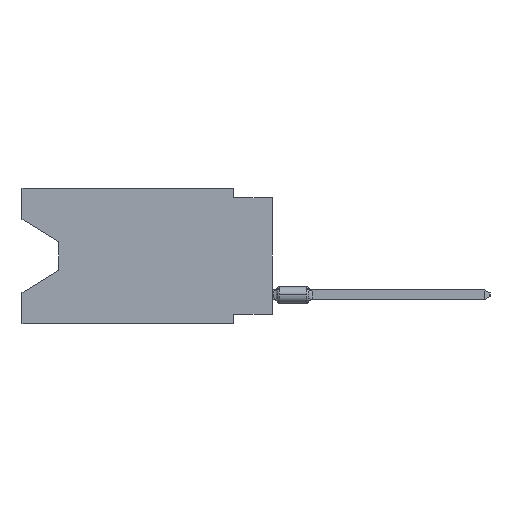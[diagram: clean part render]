
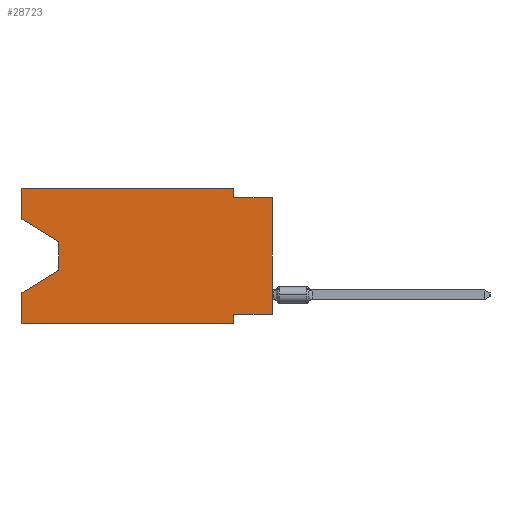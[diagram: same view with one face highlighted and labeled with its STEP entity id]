
A CAD part, left-side view. The second image highlights one B-rep face of the part: STEP entity #28723.
In plain terms, the highlighted planar face has unit normal (-1, 0, 0).
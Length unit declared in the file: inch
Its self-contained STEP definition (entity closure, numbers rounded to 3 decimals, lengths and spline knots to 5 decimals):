
#227 = CARTESIAN_POINT ( 'NONE',  ( 0., 0.55, -0.212 ) ) ;
#2391 = DIRECTION ( 'NONE',  ( 0., 0., -1. ) ) ;
#2712 = EDGE_CURVE ( 'NONE', #57532, #56211, #56468, .T. ) ;
#2886 = VERTEX_POINT ( 'NONE', #9775 ) ;
#2933 = VERTEX_POINT ( 'NONE', #9493 ) ;
#2992 = VECTOR ( 'NONE', #24589, 39.37008 ) ;
#4648 = EDGE_CURVE ( 'NONE', #56844, #14403, #43599, .T. ) ;
#4980 = LINE ( 'NONE', #18821, #54229 ) ;
#5857 = DIRECTION ( 'NONE',  ( 0., 0., -1. ) ) ;
#6178 = ORIENTED_EDGE ( 'NONE', *, *, #4648, .F. ) ;
#6564 = ORIENTED_EDGE ( 'NONE', *, *, #32936, .T. ) ;
#8254 = ORIENTED_EDGE ( 'NONE', *, *, #43584, .F. ) ;
#8475 = LINE ( 'NONE', #18488, #22472 ) ;
#8972 = VECTOR ( 'NONE', #2391, 39.37008 ) ;
#9493 = CARTESIAN_POINT ( 'NONE',  ( 0., 0.1, -0.35 ) ) ;
#9775 = CARTESIAN_POINT ( 'NONE',  ( 0., 0.55, -0.212 ) ) ;
#9918 = DIRECTION ( 'NONE',  ( 0., 0., -1. ) ) ;
#10301 = CARTESIAN_POINT ( 'NONE',  ( 0., 0.645, -0.35 ) ) ;
#11115 = VERTEX_POINT ( 'NONE', #48294 ) ;
#11259 = CARTESIAN_POINT ( 'NONE',  ( 0., 0.645, 0. ) ) ;
#12315 = DIRECTION ( 'NONE',  ( 0., 0., 1. ) ) ;
#12634 = VERTEX_POINT ( 'NONE', #15781 ) ;
#13958 = DIRECTION ( 'NONE',  ( 0., 0., 1. ) ) ;
#14261 = LINE ( 'NONE', #44655, #40225 ) ;
#14403 = VERTEX_POINT ( 'NONE', #43560 ) ;
#15482 = VERTEX_POINT ( 'NONE', #50752 ) ;
#15781 = CARTESIAN_POINT ( 'NONE',  ( 0., 0.645, -0.08025 ) ) ;
#16506 = VECTOR ( 'NONE', #22323, 39.37008 ) ;
#17319 = CARTESIAN_POINT ( 'NONE',  ( 0., 0.1, -0.35 ) ) ;
#17358 = ORIENTED_EDGE ( 'NONE', *, *, #53303, .T. ) ;
#17452 = ORIENTED_EDGE ( 'NONE', *, *, #23406, .T. ) ;
#17510 = CARTESIAN_POINT ( 'NONE',  ( 0., 0., -0.025 ) ) ;
#17907 = FACE_OUTER_BOUND ( 'NONE', #54337, .T. ) ;
#18488 = CARTESIAN_POINT ( 'NONE',  ( 0., 0.645, -0.35 ) ) ;
#18821 = CARTESIAN_POINT ( 'NONE',  ( 0., 0.1, 0. ) ) ;
#19111 = VERTEX_POINT ( 'NONE', #30902 ) ;
#19414 = CARTESIAN_POINT ( 'NONE',  ( 0., 0.645, 0. ) ) ;
#19599 = ORIENTED_EDGE ( 'NONE', *, *, #25266, .T. ) ;
#19929 = EDGE_CURVE ( 'NONE', #2886, #14403, #36800, .T. ) ;
#20009 = ORIENTED_EDGE ( 'NONE', *, *, #57315, .F. ) ;
#20077 = EDGE_CURVE ( 'NONE', #12634, #45940, #25446, .T. ) ;
#21761 = LINE ( 'NONE', #22044, #16506 ) ;
#21843 = ORIENTED_EDGE ( 'NONE', *, *, #39135, .F. ) ;
#22044 = CARTESIAN_POINT ( 'NONE',  ( 0., 0.645, -0.08025 ) ) ;
#22323 = DIRECTION ( 'NONE',  ( 0., -0.855, -0.519 ) ) ;
#22472 = VECTOR ( 'NONE', #22630, 39.37008 ) ;
#22624 = DIRECTION ( 'NONE',  ( 0., 0.855, -0.519 ) ) ;
#22630 = DIRECTION ( 'NONE',  ( 0., -1., 0. ) ) ;
#22679 = DIRECTION ( 'NONE',  ( 0., -1., 0. ) ) ;
#23406 = EDGE_CURVE ( 'NONE', #57532, #36121, #14261, .T. ) ;
#24589 = DIRECTION ( 'NONE',  ( 0., 0., 1. ) ) ;
#25266 = EDGE_CURVE ( 'NONE', #56844, #2933, #8475, .T. ) ;
#25446 = LINE ( 'NONE', #38750, #2992 ) ;
#26273 = CARTESIAN_POINT ( 'NONE',  ( 0., 0.55, -0.138 ) ) ;
#26746 = DIRECTION ( 'NONE',  ( 1., 0., 0. ) ) ;
#26839 = DIRECTION ( 'NONE',  ( 0., 0., -1. ) ) ;
#27221 = VECTOR ( 'NONE', #12315, 39.37008 ) ;
#28723 = ADVANCED_FACE ( 'NONE', ( #17907 ), #40924, .F. ) ;
#28906 = ORIENTED_EDGE ( 'NONE', *, *, #19929, .T. ) ;
#29237 = LINE ( 'NONE', #17319, #8972 ) ;
#30902 = CARTESIAN_POINT ( 'NONE',  ( 0., 0.1, -0.025 ) ) ;
#32936 = EDGE_CURVE ( 'NONE', #11115, #2886, #45154, .T. ) ;
#35523 = CARTESIAN_POINT ( 'NONE',  ( 0., 0., -0.025 ) ) ;
#35965 = VECTOR ( 'NONE', #22624, 39.37008 ) ;
#36121 = VERTEX_POINT ( 'NONE', #35523 ) ;
#36552 = ORIENTED_EDGE ( 'NONE', *, *, #51704, .F. ) ;
#36701 = CARTESIAN_POINT ( 'NONE',  ( 0., 0., -0.325 ) ) ;
#36800 = LINE ( 'NONE', #227, #35965 ) ;
#36855 = LINE ( 'NONE', #19414, #42419 ) ;
#37038 = CARTESIAN_POINT ( 'NONE',  ( 0., 0.1, -0.325 ) ) ;
#38750 = CARTESIAN_POINT ( 'NONE',  ( 0., 0.645, 0. ) ) ;
#39135 = EDGE_CURVE ( 'NONE', #56211, #2933, #29237, .T. ) ;
#40225 = VECTOR ( 'NONE', #13958, 39.37008 ) ;
#40407 = VECTOR ( 'NONE', #57326, 39.37008 ) ;
#40924 = PLANE ( 'NONE',  #53612 ) ;
#42419 = VECTOR ( 'NONE', #22679, 39.37008 ) ;
#43560 = CARTESIAN_POINT ( 'NONE',  ( 0., 0.645, -0.26975 ) ) ;
#43584 = EDGE_CURVE ( 'NONE', #45940, #15482, #36855, .T. ) ;
#43599 = LINE ( 'NONE', #48604, #27221 ) ;
#44077 = LINE ( 'NONE', #17510, #45969 ) ;
#44491 = ORIENTED_EDGE ( 'NONE', *, *, #2712, .F. ) ;
#44655 = CARTESIAN_POINT ( 'NONE',  ( 0., 0., 0. ) ) ;
#45154 = LINE ( 'NONE', #26273, #54766 ) ;
#45940 = VERTEX_POINT ( 'NONE', #11259 ) ;
#45969 = VECTOR ( 'NONE', #49105, 39.37008 ) ;
#48294 = CARTESIAN_POINT ( 'NONE',  ( 0., 0.55, -0.138 ) ) ;
#48604 = CARTESIAN_POINT ( 'NONE',  ( 0., 0.645, 0. ) ) ;
#49105 = DIRECTION ( 'NONE',  ( 0., -1., 0. ) ) ;
#49561 = ORIENTED_EDGE ( 'NONE', *, *, #20077, .F. ) ;
#50752 = CARTESIAN_POINT ( 'NONE',  ( 0., 0.1, 0. ) ) ;
#51704 = EDGE_CURVE ( 'NONE', #15482, #19111, #4980, .T. ) ;
#52033 = CARTESIAN_POINT ( 'NONE',  ( 0., 0., -0.325 ) ) ;
#53303 = EDGE_CURVE ( 'NONE', #12634, #11115, #21761, .T. ) ;
#53612 = AXIS2_PLACEMENT_3D ( 'NONE', #54795, #26746, #9918 ) ;
#54229 = VECTOR ( 'NONE', #5857, 39.37008 ) ;
#54337 = EDGE_LOOP ( 'NONE', ( #17358, #6564, #28906, #6178, #19599, #21843, #44491, #17452, #20009, #36552, #8254, #49561 ) ) ;
#54766 = VECTOR ( 'NONE', #26839, 39.37008 ) ;
#54795 = CARTESIAN_POINT ( 'NONE',  ( 0., 0.645, 0. ) ) ;
#56211 = VERTEX_POINT ( 'NONE', #37038 ) ;
#56468 = LINE ( 'NONE', #52033, #40407 ) ;
#56844 = VERTEX_POINT ( 'NONE', #10301 ) ;
#57315 = EDGE_CURVE ( 'NONE', #19111, #36121, #44077, .T. ) ;
#57326 = DIRECTION ( 'NONE',  ( 0., 1., 0. ) ) ;
#57532 = VERTEX_POINT ( 'NONE', #36701 ) ;
